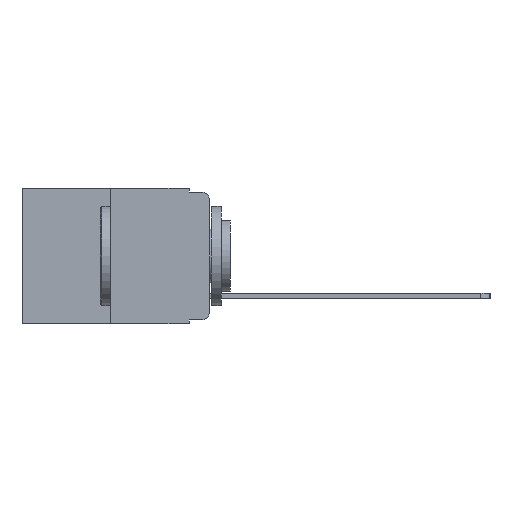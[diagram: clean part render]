
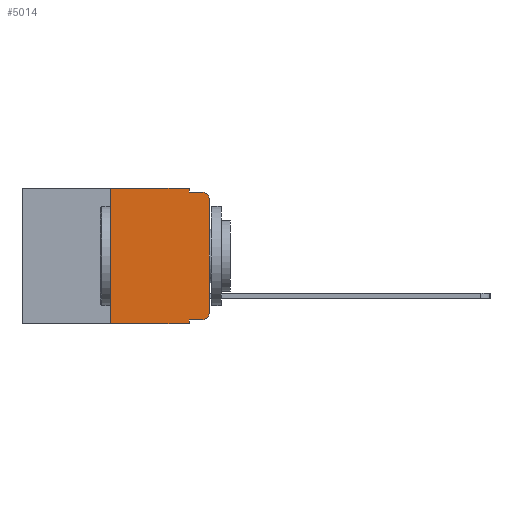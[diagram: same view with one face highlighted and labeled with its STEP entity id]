
A CAD part, left-side view. The second image highlights one B-rep face of the part: STEP entity #5014.
In plain terms, the highlighted planar face has unit normal (-1, 0, 0).
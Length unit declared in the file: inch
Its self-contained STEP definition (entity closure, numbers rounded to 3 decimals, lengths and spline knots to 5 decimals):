
#39 = CARTESIAN_POINT ( 'NONE',  ( 0., 0., -0.313 ) ) ;
#49 = ORIENTED_EDGE ( 'NONE', *, *, #8726, .F. ) ;
#210 = ORIENTED_EDGE ( 'NONE', *, *, #7591, .F. ) ;
#284 = FACE_OUTER_BOUND ( 'NONE', #12116, .T. ) ;
#809 = VERTEX_POINT ( 'NONE', #6907 ) ;
#1231 = CARTESIAN_POINT ( 'NONE',  ( 0., 0.02, -0.313 ) ) ;
#1236 = CARTESIAN_POINT ( 'NONE',  ( 0., 0.25, 0. ) ) ;
#1393 = DIRECTION ( 'NONE',  ( 0., -1., 0. ) ) ;
#1587 = ORIENTED_EDGE ( 'NONE', *, *, #1821, .T. ) ;
#1716 = LINE ( 'NONE', #1236, #9555 ) ;
#1762 = VECTOR ( 'NONE', #7963, 39.37008 ) ;
#1821 = EDGE_CURVE ( 'NONE', #809, #2476, #10328, .T. ) ;
#2367 = DIRECTION ( 'NONE',  ( 0., 0., 1. ) ) ;
#2476 = VERTEX_POINT ( 'NONE', #39 ) ;
#2697 = ORIENTED_EDGE ( 'NONE', *, *, #11988, .T. ) ;
#2884 = CARTESIAN_POINT ( 'NONE',  ( 0., 0.051, -0.01 ) ) ;
#3033 = DIRECTION ( 'NONE',  ( 0., 0., -1. ) ) ;
#3211 = ORIENTED_EDGE ( 'NONE', *, *, #4002, .T. ) ;
#3423 = CARTESIAN_POINT ( 'NONE',  ( 0., 0.051, 0. ) ) ;
#4002 = EDGE_CURVE ( 'NONE', #6908, #809, #4652, .T. ) ;
#4296 = CARTESIAN_POINT ( 'NONE',  ( 0., 0.051, -0.333 ) ) ;
#4652 = LINE ( 'NONE', #4296, #1762 ) ;
#4722 = VERTEX_POINT ( 'NONE', #6359 ) ;
#4735 = VECTOR ( 'NONE', #1393, 39.37008 ) ;
#4739 = VERTEX_POINT ( 'NONE', #12976 ) ;
#4793 = CARTESIAN_POINT ( 'NONE',  ( 0., 0.051, -0.01 ) ) ;
#5014 = ADVANCED_FACE ( 'NONE', ( #284 ), #9612, .F. ) ;
#5122 = EDGE_CURVE ( 'NONE', #2476, #4722, #8107, .T. ) ;
#5388 = ORIENTED_EDGE ( 'NONE', *, *, #8990, .T. ) ;
#5567 = VECTOR ( 'NONE', #11236, 39.37008 ) ;
#5571 = CIRCLE ( 'NONE', #8479, 0.02 ) ;
#5795 = CARTESIAN_POINT ( 'NONE',  ( 0., 0.02, -0.03 ) ) ;
#6063 = AXIS2_PLACEMENT_3D ( 'NONE', #1231, #9992, #9711 ) ;
#6359 = CARTESIAN_POINT ( 'NONE',  ( 0., 0., -0.03 ) ) ;
#6514 = CARTESIAN_POINT ( 'NONE',  ( 0., 0.473, -0.343 ) ) ;
#6552 = AXIS2_PLACEMENT_3D ( 'NONE', #12323, #12456, #12397 ) ;
#6858 = DIRECTION ( 'NONE',  ( 0., 0., -1. ) ) ;
#6875 = ORIENTED_EDGE ( 'NONE', *, *, #11631, .F. ) ;
#6907 = CARTESIAN_POINT ( 'NONE',  ( 0., 0.02, -0.333 ) ) ;
#6908 = VERTEX_POINT ( 'NONE', #10185 ) ;
#7179 = DIRECTION ( 'NONE',  ( 0., -1., 0. ) ) ;
#7204 = CARTESIAN_POINT ( 'NONE',  ( 0., 0.051, 0. ) ) ;
#7530 = LINE ( 'NONE', #2884, #9937 ) ;
#7564 = LINE ( 'NONE', #10368, #12472 ) ;
#7588 = DIRECTION ( 'NONE',  ( 0., -1., 0. ) ) ;
#7591 = EDGE_CURVE ( 'NONE', #6908, #4739, #11628, .T. ) ;
#7892 = CARTESIAN_POINT ( 'NONE',  ( 0., 0.25, -0.343 ) ) ;
#7897 = LINE ( 'NONE', #9905, #4735 ) ;
#7963 = DIRECTION ( 'NONE',  ( 0., -1., 0. ) ) ;
#8020 = VERTEX_POINT ( 'NONE', #7892 ) ;
#8035 = CARTESIAN_POINT ( 'NONE',  ( 0., 0.02, -0.01 ) ) ;
#8107 = LINE ( 'NONE', #9867, #10805 ) ;
#8479 = AXIS2_PLACEMENT_3D ( 'NONE', #5795, #12782, #6858 ) ;
#8726 = EDGE_CURVE ( 'NONE', #13118, #9353, #7530, .T. ) ;
#8990 = EDGE_CURVE ( 'NONE', #8020, #4739, #12293, .T. ) ;
#9058 = VERTEX_POINT ( 'NONE', #3423 ) ;
#9353 = VERTEX_POINT ( 'NONE', #8035 ) ;
#9473 = VECTOR ( 'NONE', #7588, 39.37008 ) ;
#9555 = VECTOR ( 'NONE', #2367, 39.37008 ) ;
#9612 = PLANE ( 'NONE',  #6552 ) ;
#9711 = DIRECTION ( 'NONE',  ( 0., 0., -1. ) ) ;
#9867 = CARTESIAN_POINT ( 'NONE',  ( 0., 0., 0. ) ) ;
#9905 = CARTESIAN_POINT ( 'NONE',  ( 0., 0.473, 0. ) ) ;
#9937 = VECTOR ( 'NONE', #7179, 39.37008 ) ;
#9952 = ORIENTED_EDGE ( 'NONE', *, *, #10334, .F. ) ;
#9992 = DIRECTION ( 'NONE',  ( -1., 0., 0. ) ) ;
#10185 = CARTESIAN_POINT ( 'NONE',  ( 0., 0.051, -0.333 ) ) ;
#10328 = CIRCLE ( 'NONE', #6063, 0.02 ) ;
#10334 = EDGE_CURVE ( 'NONE', #8020, #13188, #1716, .T. ) ;
#10368 = CARTESIAN_POINT ( 'NONE',  ( 0., 0.051, 0. ) ) ;
#10530 = DIRECTION ( 'NONE',  ( 0., 0., 1. ) ) ;
#10805 = VECTOR ( 'NONE', #10530, 39.37008 ) ;
#11236 = DIRECTION ( 'NONE',  ( 0., 0., -1. ) ) ;
#11610 = ORIENTED_EDGE ( 'NONE', *, *, #12207, .F. ) ;
#11628 = LINE ( 'NONE', #7204, #5567 ) ;
#11631 = EDGE_CURVE ( 'NONE', #13188, #9058, #7897, .T. ) ;
#11988 = EDGE_CURVE ( 'NONE', #4722, #9353, #5571, .T. ) ;
#12116 = EDGE_LOOP ( 'NONE', ( #13173, #2697, #49, #11610, #6875, #9952, #5388, #210, #3211, #1587 ) ) ;
#12207 = EDGE_CURVE ( 'NONE', #9058, #13118, #7564, .T. ) ;
#12293 = LINE ( 'NONE', #6514, #9473 ) ;
#12323 = CARTESIAN_POINT ( 'NONE',  ( 0., 0.473, 0. ) ) ;
#12397 = DIRECTION ( 'NONE',  ( 0., 0., -1. ) ) ;
#12456 = DIRECTION ( 'NONE',  ( 1., 0., 0. ) ) ;
#12472 = VECTOR ( 'NONE', #3033, 39.37008 ) ;
#12782 = DIRECTION ( 'NONE',  ( -1., 0., 0. ) ) ;
#12900 = CARTESIAN_POINT ( 'NONE',  ( 0., 0.25, 0. ) ) ;
#12976 = CARTESIAN_POINT ( 'NONE',  ( 0., 0.051, -0.343 ) ) ;
#13118 = VERTEX_POINT ( 'NONE', #4793 ) ;
#13173 = ORIENTED_EDGE ( 'NONE', *, *, #5122, .T. ) ;
#13188 = VERTEX_POINT ( 'NONE', #12900 ) ;
